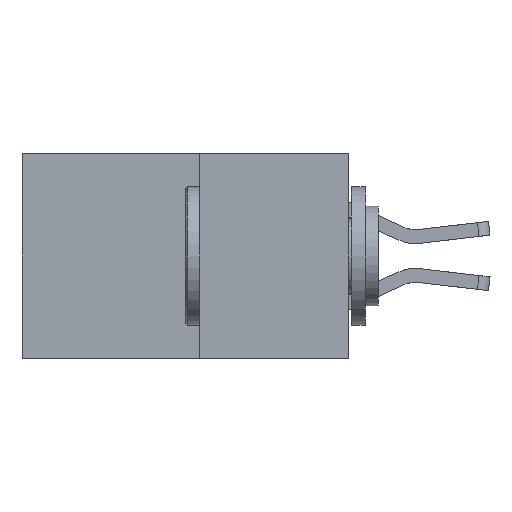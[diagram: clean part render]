
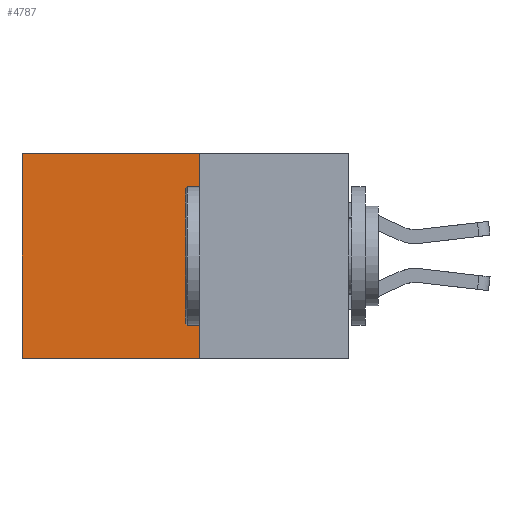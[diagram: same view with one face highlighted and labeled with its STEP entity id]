
A CAD part, left-side view. The second image highlights one B-rep face of the part: STEP entity #4787.
In plain terms, the highlighted planar face has unit normal (-1, 0, 0).
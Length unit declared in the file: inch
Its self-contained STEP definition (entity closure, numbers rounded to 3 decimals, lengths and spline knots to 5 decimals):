
#12 = VECTOR ( 'NONE', #3675, 39.37008 ) ;
#53 = EDGE_LOOP ( 'NONE', ( #3109, #6686, #3343, #8543 ) ) ;
#528 = VECTOR ( 'NONE', #7544, 39.37008 ) ;
#1094 = VERTEX_POINT ( 'NONE', #3761 ) ;
#1137 = LINE ( 'NONE', #3946, #6397 ) ;
#1159 = EDGE_CURVE ( 'NONE', #1622, #8222, #5552, .T. ) ;
#1349 = LINE ( 'NONE', #6732, #8290 ) ;
#1497 = EDGE_CURVE ( 'NONE', #1094, #8222, #1137, .T. ) ;
#1622 = VERTEX_POINT ( 'NONE', #2976 ) ;
#1706 = VERTEX_POINT ( 'NONE', #2656 ) ;
#2656 = CARTESIAN_POINT ( 'NONE',  ( 0.277, 0.27, 0. ) ) ;
#2976 = CARTESIAN_POINT ( 'NONE',  ( 0.277, 0.27, -0.37 ) ) ;
#3109 = ORIENTED_EDGE ( 'NONE', *, *, #1497, .T. ) ;
#3203 = EDGE_CURVE ( 'NONE', #1706, #1622, #1349, .T. ) ;
#3343 = ORIENTED_EDGE ( 'NONE', *, *, #3203, .F. ) ;
#3675 = DIRECTION ( 'NONE',  ( 0., 1., 0. ) ) ;
#3761 = CARTESIAN_POINT ( 'NONE',  ( 0.277, 0.59, 0. ) ) ;
#3867 = DIRECTION ( 'NONE',  ( 0., 0., -1. ) ) ;
#3946 = CARTESIAN_POINT ( 'NONE',  ( 0.277, 0.59, -0.37 ) ) ;
#4607 = FACE_OUTER_BOUND ( 'NONE', #53, .T. ) ;
#4787 = ADVANCED_FACE ( 'NONE', ( #4607 ), #8050, .F. ) ;
#5267 = EDGE_CURVE ( 'NONE', #1706, #1094, #6056, .T. ) ;
#5552 = LINE ( 'NONE', #6542, #12 ) ;
#6056 = LINE ( 'NONE', #7602, #528 ) ;
#6397 = VECTOR ( 'NONE', #7476, 39.37008 ) ;
#6542 = CARTESIAN_POINT ( 'NONE',  ( 0.277, 0.27, -0.37 ) ) ;
#6686 = ORIENTED_EDGE ( 'NONE', *, *, #1159, .F. ) ;
#6732 = CARTESIAN_POINT ( 'NONE',  ( 0.277, 0.27, -0.37 ) ) ;
#7476 = DIRECTION ( 'NONE',  ( 0., 0., -1. ) ) ;
#7544 = DIRECTION ( 'NONE',  ( 0., 1., 0. ) ) ;
#7602 = CARTESIAN_POINT ( 'NONE',  ( 0.277, 0.27, 0. ) ) ;
#7606 = CARTESIAN_POINT ( 'NONE',  ( 0.277, 0.59, -0.37 ) ) ;
#7739 = DIRECTION ( 'NONE',  ( 1., 0., 0. ) ) ;
#7760 = CARTESIAN_POINT ( 'NONE',  ( 0.277, 0.27, -0.37 ) ) ;
#7785 = DIRECTION ( 'NONE',  ( 0., 0., -1. ) ) ;
#8050 = PLANE ( 'NONE',  #8383 ) ;
#8222 = VERTEX_POINT ( 'NONE', #7606 ) ;
#8290 = VECTOR ( 'NONE', #3867, 39.37008 ) ;
#8383 = AXIS2_PLACEMENT_3D ( 'NONE', #7760, #7739, #7785 ) ;
#8543 = ORIENTED_EDGE ( 'NONE', *, *, #5267, .T. ) ;
